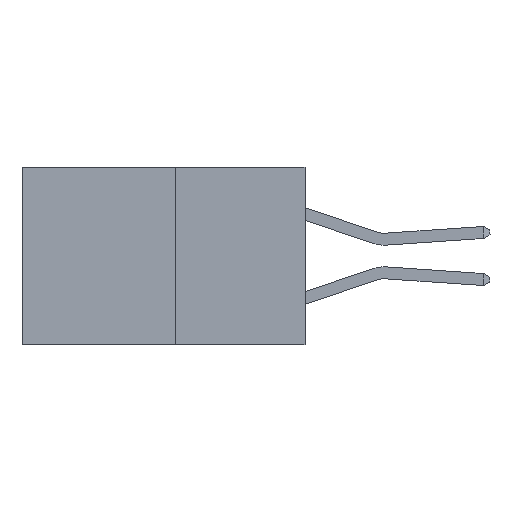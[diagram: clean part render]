
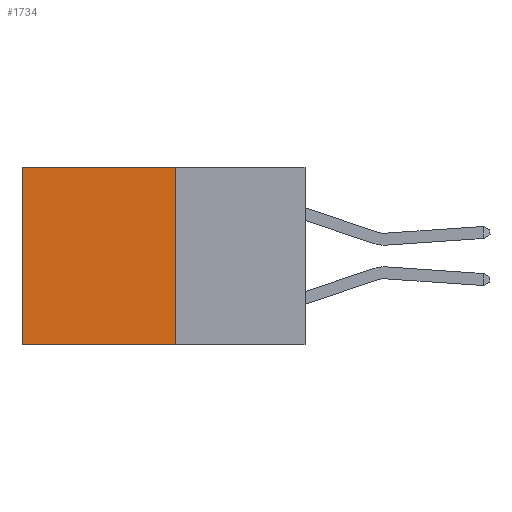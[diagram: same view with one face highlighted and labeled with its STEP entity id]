
A CAD part, left-side view. The second image highlights one B-rep face of the part: STEP entity #1734.
In plain terms, the highlighted planar face has unit normal (-1, 0, 0).
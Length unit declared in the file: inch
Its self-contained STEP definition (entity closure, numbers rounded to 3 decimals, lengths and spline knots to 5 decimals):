
#133 = VECTOR ( 'NONE', #284, 39.37008 ) ;
#284 = DIRECTION ( 'NONE',  ( 0., 0., -1. ) ) ;
#760 = LINE ( 'NONE', #1515, #6503 ) ;
#893 = VECTOR ( 'NONE', #1031, 39.37008 ) ;
#1031 = DIRECTION ( 'NONE',  ( 0., 0., -1. ) ) ;
#1055 = VERTEX_POINT ( 'NONE', #9141 ) ;
#1515 = CARTESIAN_POINT ( 'NONE',  ( 0.277, 0.27, 0. ) ) ;
#1617 = CARTESIAN_POINT ( 'NONE',  ( 0.277, 0.27, -0.37 ) ) ;
#1734 = ADVANCED_FACE ( 'NONE', ( #8076 ), #7742, .F. ) ;
#1818 = AXIS2_PLACEMENT_3D ( 'NONE', #3048, #2971, #5267 ) ;
#2324 = ORIENTED_EDGE ( 'NONE', *, *, #7361, .F. ) ;
#2971 = DIRECTION ( 'NONE',  ( 1., 0., 0. ) ) ;
#3048 = CARTESIAN_POINT ( 'NONE',  ( 0.277, 0.27, -0.37 ) ) ;
#3136 = VERTEX_POINT ( 'NONE', #9095 ) ;
#4014 = VERTEX_POINT ( 'NONE', #8620 ) ;
#4066 = ORIENTED_EDGE ( 'NONE', *, *, #7463, .T. ) ;
#4207 = DIRECTION ( 'NONE',  ( 0., 1., 0. ) ) ;
#4216 = LINE ( 'NONE', #6299, #133 ) ;
#4285 = ORIENTED_EDGE ( 'NONE', *, *, #9482, .T. ) ;
#4500 = CARTESIAN_POINT ( 'NONE',  ( 0.277, 0.27, -0.37 ) ) ;
#4992 = EDGE_LOOP ( 'NONE', ( #4066, #7942, #2324, #4285 ) ) ;
#5213 = DIRECTION ( 'NONE',  ( 0., 1., 0. ) ) ;
#5267 = DIRECTION ( 'NONE',  ( 0., 0., -1. ) ) ;
#6175 = VECTOR ( 'NONE', #4207, 39.37008 ) ;
#6299 = CARTESIAN_POINT ( 'NONE',  ( 0.277, 0.59, -0.37 ) ) ;
#6406 = LINE ( 'NONE', #8526, #6175 ) ;
#6503 = VECTOR ( 'NONE', #5213, 39.37008 ) ;
#7361 = EDGE_CURVE ( 'NONE', #3136, #7889, #8703, .T. ) ;
#7463 = EDGE_CURVE ( 'NONE', #1055, #4014, #4216, .T. ) ;
#7742 = PLANE ( 'NONE',  #1818 ) ;
#7889 = VERTEX_POINT ( 'NONE', #4500 ) ;
#7942 = ORIENTED_EDGE ( 'NONE', *, *, #8357, .F. ) ;
#8076 = FACE_OUTER_BOUND ( 'NONE', #4992, .T. ) ;
#8357 = EDGE_CURVE ( 'NONE', #7889, #4014, #6406, .T. ) ;
#8526 = CARTESIAN_POINT ( 'NONE',  ( 0.277, 0.27, -0.37 ) ) ;
#8620 = CARTESIAN_POINT ( 'NONE',  ( 0.277, 0.59, -0.37 ) ) ;
#8703 = LINE ( 'NONE', #1617, #893 ) ;
#9095 = CARTESIAN_POINT ( 'NONE',  ( 0.277, 0.27, 0. ) ) ;
#9141 = CARTESIAN_POINT ( 'NONE',  ( 0.277, 0.59, 0. ) ) ;
#9482 = EDGE_CURVE ( 'NONE', #3136, #1055, #760, .T. ) ;
